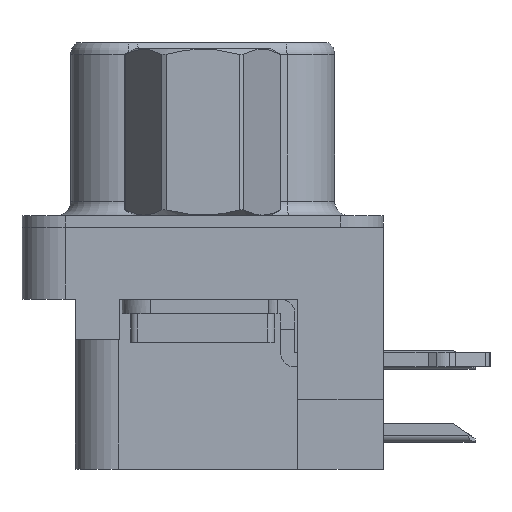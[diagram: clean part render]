
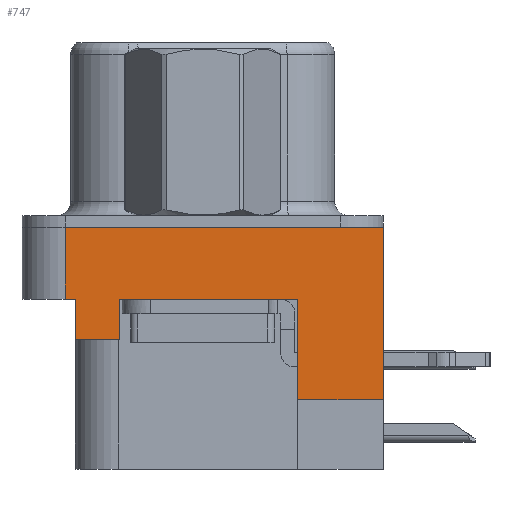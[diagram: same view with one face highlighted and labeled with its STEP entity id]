
A CAD part, left-side view. The second image highlights one B-rep face of the part: STEP entity #747.
In plain terms, the highlighted planar face has unit normal (-1, 0, 0).
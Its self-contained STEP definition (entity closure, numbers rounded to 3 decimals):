
#186 = EDGE_CURVE ( 'NONE', #16720, #21630, #4483, .T. ) ;
#326 = EDGE_LOOP ( 'NONE', ( #9488, #3889, #20534, #15086, #10606, #12003, #11206, #18442, #11245, #13734 ) ) ;
#465 = LINE ( 'NONE', #12670, #4821 ) ;
#702 = CARTESIAN_POINT ( 'NONE',  ( -2.935, 4.425, -3.9 ) ) ;
#740 = VERTEX_POINT ( 'NONE', #1462 ) ;
#747 = ADVANCED_FACE ( 'NONE', ( #17351 ), #1100, .T. ) ;
#756 = CARTESIAN_POINT ( 'NONE',  ( -2.935, -6.275, -2.5 ) ) ;
#917 = LINE ( 'NONE', #13977, #23663 ) ;
#1100 = PLANE ( 'NONE',  #14739 ) ;
#1146 = DIRECTION ( 'NONE',  ( 0., 1., 0. ) ) ;
#1270 = CARTESIAN_POINT ( 'NONE',  ( -2.935, -3.295, -6. ) ) ;
#1462 = CARTESIAN_POINT ( 'NONE',  ( -2.935, 2.895, -2.5 ) ) ;
#1631 = DIRECTION ( 'NONE',  ( 0., 1., 0. ) ) ;
#2011 = EDGE_CURVE ( 'NONE', #9904, #11464, #11610, .T. ) ;
#2163 = DIRECTION ( 'NONE',  ( -1., 0., 0. ) ) ;
#2181 = EDGE_CURVE ( 'NONE', #740, #16438, #3852, .T. ) ;
#2249 = CARTESIAN_POINT ( 'NONE',  ( -2.935, 4.775, -2.5 ) ) ;
#2367 = EDGE_CURVE ( 'NONE', #10441, #740, #14457, .T. ) ;
#2426 = CARTESIAN_POINT ( 'NONE',  ( -2.935, 4.775, 0. ) ) ;
#2734 = VECTOR ( 'NONE', #17257, 1000. ) ;
#2999 = CARTESIAN_POINT ( 'NONE',  ( -2.935, -6.275, -2.5 ) ) ;
#3260 = VECTOR ( 'NONE', #23144, 1000. ) ;
#3370 = LINE ( 'NONE', #15775, #22327 ) ;
#3852 = LINE ( 'NONE', #22417, #3260 ) ;
#3889 = ORIENTED_EDGE ( 'NONE', *, *, #16048, .T. ) ;
#4483 = LINE ( 'NONE', #10629, #5081 ) ;
#4821 = VECTOR ( 'NONE', #1631, 1000. ) ;
#4922 = CARTESIAN_POINT ( 'NONE',  ( -2.935, 2.895, -3.9 ) ) ;
#4977 = DIRECTION ( 'NONE',  ( 0., 0., 1. ) ) ;
#5081 = VECTOR ( 'NONE', #15418, 1000. ) ;
#5841 = CARTESIAN_POINT ( 'NONE',  ( -2.935, 2.895, -3.9 ) ) ;
#6201 = VECTOR ( 'NONE', #11848, 1000. ) ;
#7689 = LINE ( 'NONE', #702, #2734 ) ;
#8013 = VERTEX_POINT ( 'NONE', #8600 ) ;
#8600 = CARTESIAN_POINT ( 'NONE',  ( -2.935, 4.425, -3.9 ) ) ;
#9078 = CARTESIAN_POINT ( 'NONE',  ( -2.935, -6.275, -6. ) ) ;
#9488 = ORIENTED_EDGE ( 'NONE', *, *, #16181, .F. ) ;
#9904 = VERTEX_POINT ( 'NONE', #17768 ) ;
#10002 = VECTOR ( 'NONE', #11783, 1000. ) ;
#10019 = LINE ( 'NONE', #2249, #18626 ) ;
#10024 = CARTESIAN_POINT ( 'NONE',  ( -2.935, -6.275, -2.5 ) ) ;
#10182 = VECTOR ( 'NONE', #20340, 1000. ) ;
#10441 = VERTEX_POINT ( 'NONE', #4922 ) ;
#10606 = ORIENTED_EDGE ( 'NONE', *, *, #2011, .T. ) ;
#10629 = CARTESIAN_POINT ( 'NONE',  ( -2.935, -6.275, 0. ) ) ;
#11206 = ORIENTED_EDGE ( 'NONE', *, *, #16373, .F. ) ;
#11245 = ORIENTED_EDGE ( 'NONE', *, *, #2181, .T. ) ;
#11299 = EDGE_CURVE ( 'NONE', #9904, #16720, #10019, .T. ) ;
#11464 = VERTEX_POINT ( 'NONE', #21377 ) ;
#11610 = LINE ( 'NONE', #10024, #6201 ) ;
#11783 = DIRECTION ( 'NONE',  ( 0., 0., 1. ) ) ;
#11848 = DIRECTION ( 'NONE',  ( 0., -1., 0. ) ) ;
#12003 = ORIENTED_EDGE ( 'NONE', *, *, #17425, .F. ) ;
#12670 = CARTESIAN_POINT ( 'NONE',  ( -2.935, 4.425, -3.9 ) ) ;
#13734 = ORIENTED_EDGE ( 'NONE', *, *, #20386, .F. ) ;
#13977 = CARTESIAN_POINT ( 'NONE',  ( -2.935, -3.295, -8.4 ) ) ;
#14239 = VERTEX_POINT ( 'NONE', #9078 ) ;
#14457 = LINE ( 'NONE', #5841, #10182 ) ;
#14677 = VERTEX_POINT ( 'NONE', #1270 ) ;
#14739 = AXIS2_PLACEMENT_3D ( 'NONE', #2999, #2163, #4977 ) ;
#14865 = LINE ( 'NONE', #756, #10002 ) ;
#15086 = ORIENTED_EDGE ( 'NONE', *, *, #11299, .F. ) ;
#15418 = DIRECTION ( 'NONE',  ( 0., -1., 0. ) ) ;
#15775 = CARTESIAN_POINT ( 'NONE',  ( -2.935, -6.495, -6. ) ) ;
#16048 = EDGE_CURVE ( 'NONE', #14239, #21630, #14865, .T. ) ;
#16181 = EDGE_CURVE ( 'NONE', #14239, #14677, #3370, .T. ) ;
#16373 = EDGE_CURVE ( 'NONE', #10441, #8013, #465, .T. ) ;
#16438 = VERTEX_POINT ( 'NONE', #20147 ) ;
#16720 = VERTEX_POINT ( 'NONE', #2426 ) ;
#16950 = DIRECTION ( 'NONE',  ( 0., 0., 1. ) ) ;
#17257 = DIRECTION ( 'NONE',  ( 0., 0., 1. ) ) ;
#17351 = FACE_OUTER_BOUND ( 'NONE', #326, .T. ) ;
#17425 = EDGE_CURVE ( 'NONE', #8013, #11464, #7689, .T. ) ;
#17768 = CARTESIAN_POINT ( 'NONE',  ( -2.935, 4.775, -2.5 ) ) ;
#18442 = ORIENTED_EDGE ( 'NONE', *, *, #2367, .T. ) ;
#18626 = VECTOR ( 'NONE', #16950, 1000. ) ;
#20147 = CARTESIAN_POINT ( 'NONE',  ( -2.935, -3.295, -2.5 ) ) ;
#20340 = DIRECTION ( 'NONE',  ( 0., 0., 1. ) ) ;
#20386 = EDGE_CURVE ( 'NONE', #14677, #16438, #917, .T. ) ;
#20534 = ORIENTED_EDGE ( 'NONE', *, *, #186, .F. ) ;
#21300 = DIRECTION ( 'NONE',  ( 0., 0., 1. ) ) ;
#21377 = CARTESIAN_POINT ( 'NONE',  ( -2.935, 4.425, -2.5 ) ) ;
#21630 = VERTEX_POINT ( 'NONE', #22936 ) ;
#22327 = VECTOR ( 'NONE', #1146, 1000. ) ;
#22417 = CARTESIAN_POINT ( 'NONE',  ( -2.935, -6.275, -2.5 ) ) ;
#22936 = CARTESIAN_POINT ( 'NONE',  ( -2.935, -6.275, 0. ) ) ;
#23144 = DIRECTION ( 'NONE',  ( 0., -1., 0. ) ) ;
#23663 = VECTOR ( 'NONE', #21300, 1000. ) ;
